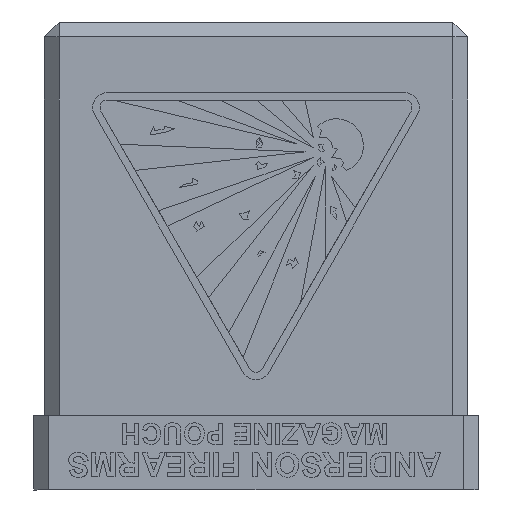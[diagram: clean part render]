
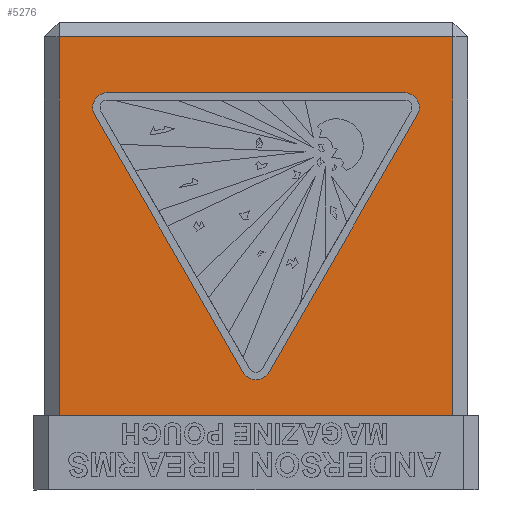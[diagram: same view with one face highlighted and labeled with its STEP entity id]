
A CAD part, front view. The second image highlights one B-rep face of the part: STEP entity #5276.
In plain terms, the highlighted planar face has unit normal (0, -1, 0).
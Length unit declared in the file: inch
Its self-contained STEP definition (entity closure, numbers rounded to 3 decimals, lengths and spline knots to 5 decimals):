
#636 = VECTOR ( 'NONE', #32282, 39.37008 ) ;
#654 = EDGE_LOOP ( 'NONE', ( #24512, #5668, #33735, #39730 ) ) ;
#668 = ORIENTED_EDGE ( 'NONE', *, *, #32718, .F. ) ;
#1504 = DIRECTION ( 'NONE',  ( 0., 0., 1. ) ) ;
#2703 = CARTESIAN_POINT ( 'NONE',  ( 1.325, -0.72929, 2.9 ) ) ;
#3146 = DIRECTION ( 'NONE',  ( 0., -1., 0. ) ) ;
#3213 = LINE ( 'NONE', #21357, #34281 ) ;
#4652 = ORIENTED_EDGE ( 'NONE', *, *, #45803, .F. ) ;
#4984 = VECTOR ( 'NONE', #10559, 39.37008 ) ;
#5276 = ADVANCED_FACE ( 'NONE', ( #37707, #27170 ), #25035, .F. ) ;
#5668 = ORIENTED_EDGE ( 'NONE', *, *, #45471, .T. ) ;
#7483 = CARTESIAN_POINT ( 'NONE',  ( -1.425, -0.72929, 0.1 ) ) ;
#7607 = ORIENTED_EDGE ( 'NONE', *, *, #36148, .F. ) ;
#7866 = LINE ( 'NONE', #32032, #27275 ) ;
#10559 = DIRECTION ( 'NONE',  ( 0.5, 0., -0.866 ) ) ;
#10677 = DIRECTION ( 'NONE',  ( 0.5, 0., 0.866 ) ) ;
#11327 = AXIS2_PLACEMENT_3D ( 'NONE', #33451, #22735, #1504 ) ;
#11339 = CARTESIAN_POINT ( 'NONE',  ( -1.325, -0.72929, 2.9 ) ) ;
#11383 = CARTESIAN_POINT ( 'NONE',  ( 1., -0.72929, 2.525 ) ) ;
#11884 = DIRECTION ( 'NONE',  ( 0., 0., -1. ) ) ;
#12692 = CARTESIAN_POINT ( 'NONE',  ( 0.0866, -0.72929, 0.64295 ) ) ;
#12768 = CARTESIAN_POINT ( 'NONE',  ( 1., -0.72929, 2.425 ) ) ;
#14110 = CARTESIAN_POINT ( 'NONE',  ( -1.325, -0.72929, 0.35 ) ) ;
#14426 = LINE ( 'NONE', #31772, #4984 ) ;
#14734 = CIRCLE ( 'NONE', #11327, 0.1 ) ;
#15372 = VERTEX_POINT ( 'NONE', #40300 ) ;
#15650 = EDGE_CURVE ( 'NONE', #25396, #33111, #31892, .T. ) ;
#15753 = VECTOR ( 'NONE', #11884, 39.37008 ) ;
#16007 = EDGE_LOOP ( 'NONE', ( #4652, #29703, #45285, #7607, #42410, #668 ) ) ;
#16329 = CIRCLE ( 'NONE', #26193, 0.1 ) ;
#16403 = VERTEX_POINT ( 'NONE', #30295 ) ;
#17487 = DIRECTION ( 'NONE',  ( 0., -1., 0. ) ) ;
#18992 = VERTEX_POINT ( 'NONE', #2703 ) ;
#19788 = CARTESIAN_POINT ( 'NONE',  ( -1.425, -0.72929, 0.35 ) ) ;
#19857 = VECTOR ( 'NONE', #27214, 39.37008 ) ;
#20169 = VERTEX_POINT ( 'NONE', #11383 ) ;
#20189 = LINE ( 'NONE', #36997, #15753 ) ;
#21357 = CARTESIAN_POINT ( 'NONE',  ( 1.0866, -0.72929, 2.375 ) ) ;
#21404 = VECTOR ( 'NONE', #27018, 39.37008 ) ;
#22242 = LINE ( 'NONE', #38932, #636 ) ;
#22409 = EDGE_CURVE ( 'NONE', #16403, #20169, #16329, .T. ) ;
#22735 = DIRECTION ( 'NONE',  ( 0., -1., 0. ) ) ;
#23757 = VERTEX_POINT ( 'NONE', #42752 ) ;
#23979 = AXIS2_PLACEMENT_3D ( 'NONE', #35046, #17487, #42121 ) ;
#24203 = EDGE_CURVE ( 'NONE', #18992, #27847, #7866, .T. ) ;
#24512 = ORIENTED_EDGE ( 'NONE', *, *, #43737, .T. ) ;
#24538 = DIRECTION ( 'NONE',  ( 0., 0., -1. ) ) ;
#24608 = EDGE_CURVE ( 'NONE', #20169, #15372, #22242, .T. ) ;
#25035 = PLANE ( 'NONE',  #44538 ) ;
#25396 = VERTEX_POINT ( 'NONE', #27995 ) ;
#25946 = LINE ( 'NONE', #19788, #19857 ) ;
#26193 = AXIS2_PLACEMENT_3D ( 'NONE', #12768, #3146, #24538 ) ;
#26856 = CARTESIAN_POINT ( 'NONE',  ( 1.325, -0.72929, 0.1 ) ) ;
#27018 = DIRECTION ( 'NONE',  ( 0., 0., 1. ) ) ;
#27170 = FACE_BOUND ( 'NONE', #16007, .T. ) ;
#27214 = DIRECTION ( 'NONE',  ( 1., 0., 0. ) ) ;
#27275 = VECTOR ( 'NONE', #35471, 39.37008 ) ;
#27847 = VERTEX_POINT ( 'NONE', #11339 ) ;
#27995 = CARTESIAN_POINT ( 'NONE',  ( -0.0866, -0.72929, 0.64295 ) ) ;
#29703 = ORIENTED_EDGE ( 'NONE', *, *, #24608, .F. ) ;
#30295 = CARTESIAN_POINT ( 'NONE',  ( 1.0866, -0.72929, 2.375 ) ) ;
#30823 = LINE ( 'NONE', #26856, #21404 ) ;
#31151 = VERTEX_POINT ( 'NONE', #14110 ) ;
#31626 = VERTEX_POINT ( 'NONE', #45861 ) ;
#31772 = CARTESIAN_POINT ( 'NONE',  ( -0.0866, -0.72929, 0.64295 ) ) ;
#31892 = CIRCLE ( 'NONE', #23979, 0.1 ) ;
#32032 = CARTESIAN_POINT ( 'NONE',  ( -1.425, -0.72929, 2.9 ) ) ;
#32282 = DIRECTION ( 'NONE',  ( -1., 0., 0. ) ) ;
#32458 = DIRECTION ( 'NONE',  ( 0., 1., 0. ) ) ;
#32718 = EDGE_CURVE ( 'NONE', #31626, #25396, #14426, .T. ) ;
#33111 = VERTEX_POINT ( 'NONE', #12692 ) ;
#33451 = CARTESIAN_POINT ( 'NONE',  ( -1., -0.72929, 2.425 ) ) ;
#33735 = ORIENTED_EDGE ( 'NONE', *, *, #24203, .T. ) ;
#34281 = VECTOR ( 'NONE', #10677, 39.37008 ) ;
#35046 = CARTESIAN_POINT ( 'NONE',  ( 0., -0.72929, 0.69295 ) ) ;
#35471 = DIRECTION ( 'NONE',  ( -1., 0., 0. ) ) ;
#36148 = EDGE_CURVE ( 'NONE', #33111, #16403, #3213, .T. ) ;
#36997 = CARTESIAN_POINT ( 'NONE',  ( -1.325, -0.72929, 0.1 ) ) ;
#37707 = FACE_OUTER_BOUND ( 'NONE', #654, .T. ) ;
#38774 = EDGE_CURVE ( 'NONE', #27847, #31151, #20189, .T. ) ;
#38932 = CARTESIAN_POINT ( 'NONE',  ( -1., -0.72929, 2.525 ) ) ;
#39101 = DIRECTION ( 'NONE',  ( 0., 0., 1. ) ) ;
#39730 = ORIENTED_EDGE ( 'NONE', *, *, #38774, .T. ) ;
#40300 = CARTESIAN_POINT ( 'NONE',  ( -1., -0.72929, 2.525 ) ) ;
#42121 = DIRECTION ( 'NONE',  ( 0., 0., 1. ) ) ;
#42410 = ORIENTED_EDGE ( 'NONE', *, *, #15650, .F. ) ;
#42752 = CARTESIAN_POINT ( 'NONE',  ( 1.325, -0.72929, 0.35 ) ) ;
#43737 = EDGE_CURVE ( 'NONE', #31151, #23757, #25946, .T. ) ;
#44538 = AXIS2_PLACEMENT_3D ( 'NONE', #7483, #32458, #39101 ) ;
#45285 = ORIENTED_EDGE ( 'NONE', *, *, #22409, .F. ) ;
#45471 = EDGE_CURVE ( 'NONE', #23757, #18992, #30823, .T. ) ;
#45803 = EDGE_CURVE ( 'NONE', #15372, #31626, #14734, .T. ) ;
#45861 = CARTESIAN_POINT ( 'NONE',  ( -1.0866, -0.72929, 2.375 ) ) ;
